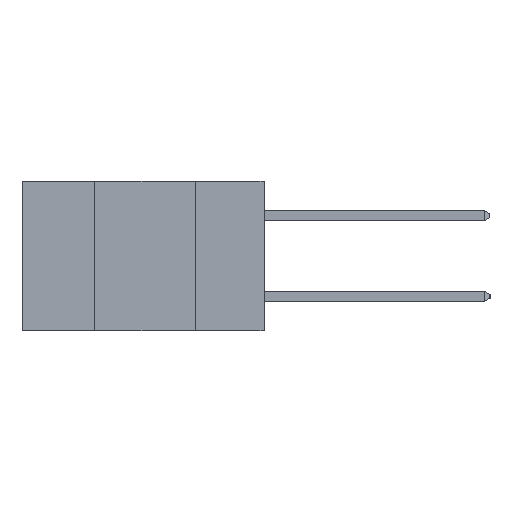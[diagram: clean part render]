
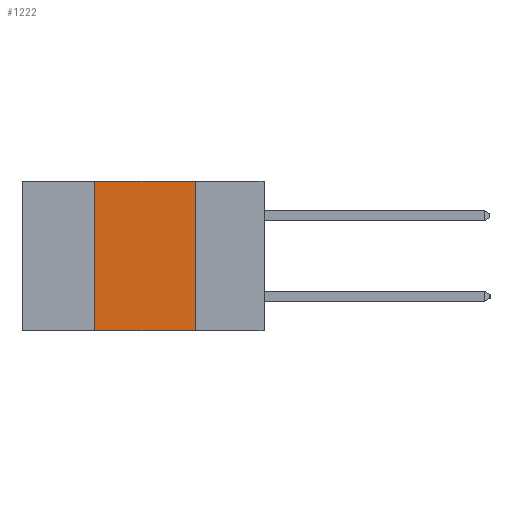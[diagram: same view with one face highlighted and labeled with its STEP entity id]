
A CAD part, left-side view. The second image highlights one B-rep face of the part: STEP entity #1222.
In plain terms, the highlighted planar face has unit normal (-1, 0, 0).
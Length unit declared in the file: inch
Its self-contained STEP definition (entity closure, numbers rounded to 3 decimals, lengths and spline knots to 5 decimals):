
#199 = ORIENTED_EDGE ( 'NONE', *, *, #13804, .T. ) ;
#1180 = VERTEX_POINT ( 'NONE', #22471 ) ;
#1202 = VERTEX_POINT ( 'NONE', #22306 ) ;
#1222 = ADVANCED_FACE ( 'NONE', ( #5990 ), #21612, .F. ) ;
#2797 = DIRECTION ( 'NONE',  ( 0., -1., 0. ) ) ;
#3547 = CARTESIAN_POINT ( 'NONE',  ( 0., 0.6, 0. ) ) ;
#3866 = CARTESIAN_POINT ( 'NONE',  ( 0., 0.42, -0.37 ) ) ;
#5470 = EDGE_CURVE ( 'NONE', #1202, #1180, #6378, .T. ) ;
#5990 = FACE_OUTER_BOUND ( 'NONE', #20519, .T. ) ;
#6378 = LINE ( 'NONE', #23094, #20952 ) ;
#8819 = EDGE_CURVE ( 'NONE', #20454, #17580, #15772, .T. ) ;
#9137 = DIRECTION ( 'NONE',  ( 0., 0., -1. ) ) ;
#9450 = DIRECTION ( 'NONE',  ( 0., 0., -1. ) ) ;
#11047 = ORIENTED_EDGE ( 'NONE', *, *, #17772, .F. ) ;
#11081 = VECTOR ( 'NONE', #2797, 39.37008 ) ;
#12326 = DIRECTION ( 'NONE',  ( 0., 0., 1. ) ) ;
#12388 = CARTESIAN_POINT ( 'NONE',  ( 0., 0.6, -0.37 ) ) ;
#13804 = EDGE_CURVE ( 'NONE', #20454, #1180, #21135, .T. ) ;
#14025 = VECTOR ( 'NONE', #18829, 39.37008 ) ;
#15501 = ORIENTED_EDGE ( 'NONE', *, *, #8819, .F. ) ;
#15772 = LINE ( 'NONE', #23669, #20769 ) ;
#17580 = VERTEX_POINT ( 'NONE', #20121 ) ;
#17695 = CARTESIAN_POINT ( 'NONE',  ( 0., 0.6, 0. ) ) ;
#17772 = EDGE_CURVE ( 'NONE', #17580, #1202, #24620, .T. ) ;
#18829 = DIRECTION ( 'NONE',  ( 0., -1., 0. ) ) ;
#19677 = AXIS2_PLACEMENT_3D ( 'NONE', #17695, #20582, #9137 ) ;
#20121 = CARTESIAN_POINT ( 'NONE',  ( 0., 0.42, 0. ) ) ;
#20454 = VERTEX_POINT ( 'NONE', #3866 ) ;
#20519 = EDGE_LOOP ( 'NONE', ( #21096, #11047, #15501, #199 ) ) ;
#20582 = DIRECTION ( 'NONE',  ( 1., 0., 0. ) ) ;
#20769 = VECTOR ( 'NONE', #12326, 39.37008 ) ;
#20952 = VECTOR ( 'NONE', #9450, 39.37008 ) ;
#21096 = ORIENTED_EDGE ( 'NONE', *, *, #5470, .F. ) ;
#21135 = LINE ( 'NONE', #12388, #11081 ) ;
#21612 = PLANE ( 'NONE',  #19677 ) ;
#22306 = CARTESIAN_POINT ( 'NONE',  ( 0., 0.17, 0. ) ) ;
#22471 = CARTESIAN_POINT ( 'NONE',  ( 0., 0.17, -0.37 ) ) ;
#23094 = CARTESIAN_POINT ( 'NONE',  ( 0., 0.17, -0.37 ) ) ;
#23669 = CARTESIAN_POINT ( 'NONE',  ( 0., 0.42, -0.37 ) ) ;
#24620 = LINE ( 'NONE', #3547, #14025 ) ;
